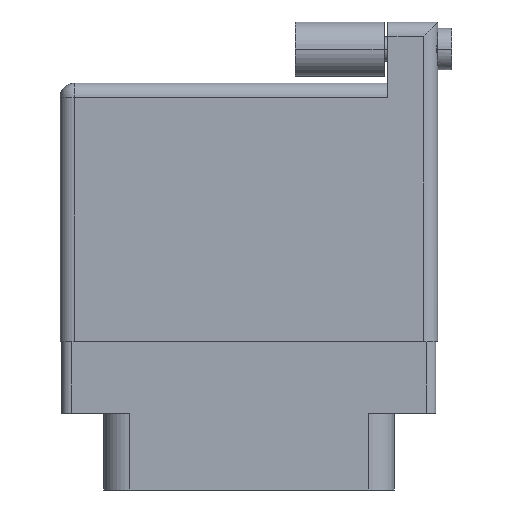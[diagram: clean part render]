
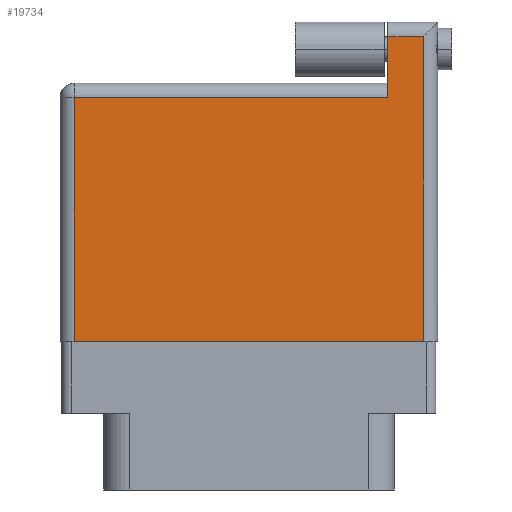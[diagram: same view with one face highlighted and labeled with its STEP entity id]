
A CAD part, front view. The second image highlights one B-rep face of the part: STEP entity #19734.
In plain terms, the highlighted face is planar.
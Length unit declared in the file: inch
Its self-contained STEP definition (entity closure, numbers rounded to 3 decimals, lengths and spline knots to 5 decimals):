
#692 = CARTESIAN_POINT ( 'NONE',  ( 1.275, 1.07, 0. ) ) ;
#1187 = LINE ( 'NONE', #18822, #2229 ) ;
#1241 = EDGE_CURVE ( 'NONE', #11290, #8816, #7864, .T. ) ;
#1488 = EDGE_LOOP ( 'NONE', ( #2196, #21095, #5416, #14540, #20127, #18246 ) ) ;
#1530 = CARTESIAN_POINT ( 'NONE',  ( 1.15, 1.07, 0. ) ) ;
#1838 = DIRECTION ( 'NONE',  ( -1., 0., 0. ) ) ;
#2131 = VERTEX_POINT ( 'NONE', #5253 ) ;
#2196 = ORIENTED_EDGE ( 'NONE', *, *, #7363, .T. ) ;
#2229 = VECTOR ( 'NONE', #8706, 39.37008 ) ;
#3410 = PLANE ( 'NONE',  #14018 ) ;
#3482 = CARTESIAN_POINT ( 'NONE',  ( 0., 1.07, 0. ) ) ;
#5253 = CARTESIAN_POINT ( 'NONE',  ( 0.05, 0.856, 0. ) ) ;
#5289 = LINE ( 'NONE', #19314, #21627 ) ;
#5416 = ORIENTED_EDGE ( 'NONE', *, *, #7259, .T. ) ;
#5662 = LINE ( 'NONE', #10792, #21974 ) ;
#6749 = LINE ( 'NONE', #14200, #11820 ) ;
#7139 = VERTEX_POINT ( 'NONE', #18586 ) ;
#7259 = EDGE_CURVE ( 'NONE', #8816, #17137, #10743, .T. ) ;
#7363 = EDGE_CURVE ( 'NONE', #14986, #11290, #5662, .T. ) ;
#7864 = LINE ( 'NONE', #14857, #12942 ) ;
#8706 = DIRECTION ( 'NONE',  ( -1., 0., 0. ) ) ;
#8816 = VERTEX_POINT ( 'NONE', #692 ) ;
#10249 = EDGE_CURVE ( 'NONE', #17137, #7139, #5289, .T. ) ;
#10743 = LINE ( 'NONE', #3482, #20401 ) ;
#10792 = CARTESIAN_POINT ( 'NONE',  ( 0., 0., 0. ) ) ;
#11290 = VERTEX_POINT ( 'NONE', #16455 ) ;
#11589 = DIRECTION ( 'NONE',  ( 0., 1., 0. ) ) ;
#11820 = VECTOR ( 'NONE', #19216, 39.37008 ) ;
#12942 = VECTOR ( 'NONE', #11589, 39.37008 ) ;
#13347 = EDGE_CURVE ( 'NONE', #2131, #14986, #6749, .T. ) ;
#13420 = DIRECTION ( 'NONE',  ( 0., 0., -1. ) ) ;
#14018 = AXIS2_PLACEMENT_3D ( 'NONE', #20470, #13420, #18519 ) ;
#14107 = CARTESIAN_POINT ( 'NONE',  ( 0.05, 0., 0. ) ) ;
#14200 = CARTESIAN_POINT ( 'NONE',  ( 0.05, 0., 0. ) ) ;
#14363 = DIRECTION ( 'NONE',  ( 1., 0., 0. ) ) ;
#14540 = ORIENTED_EDGE ( 'NONE', *, *, #10249, .T. ) ;
#14857 = CARTESIAN_POINT ( 'NONE',  ( 1.275, 1.12, 0. ) ) ;
#14986 = VERTEX_POINT ( 'NONE', #14107 ) ;
#16455 = CARTESIAN_POINT ( 'NONE',  ( 1.275, 0., 0. ) ) ;
#16667 = FACE_OUTER_BOUND ( 'NONE', #1488, .T. ) ;
#17137 = VERTEX_POINT ( 'NONE', #1530 ) ;
#18246 = ORIENTED_EDGE ( 'NONE', *, *, #13347, .T. ) ;
#18519 = DIRECTION ( 'NONE',  ( -1., 0., 0. ) ) ;
#18586 = CARTESIAN_POINT ( 'NONE',  ( 1.15, 0.856, 0. ) ) ;
#18822 = CARTESIAN_POINT ( 'NONE',  ( 0., 0.856, 0. ) ) ;
#19216 = DIRECTION ( 'NONE',  ( 0., -1., 0. ) ) ;
#19275 = EDGE_CURVE ( 'NONE', #7139, #2131, #1187, .T. ) ;
#19314 = CARTESIAN_POINT ( 'NONE',  ( 1.15, 1.12, 0. ) ) ;
#19734 = ADVANCED_FACE ( 'NONE', ( #16667 ), #3410, .F. ) ;
#20127 = ORIENTED_EDGE ( 'NONE', *, *, #19275, .T. ) ;
#20401 = VECTOR ( 'NONE', #1838, 39.37008 ) ;
#20470 = CARTESIAN_POINT ( 'NONE',  ( 0., 0.906, 0. ) ) ;
#20828 = DIRECTION ( 'NONE',  ( 0., -1., 0. ) ) ;
#21095 = ORIENTED_EDGE ( 'NONE', *, *, #1241, .T. ) ;
#21627 = VECTOR ( 'NONE', #20828, 39.37008 ) ;
#21974 = VECTOR ( 'NONE', #14363, 39.37008 ) ;
